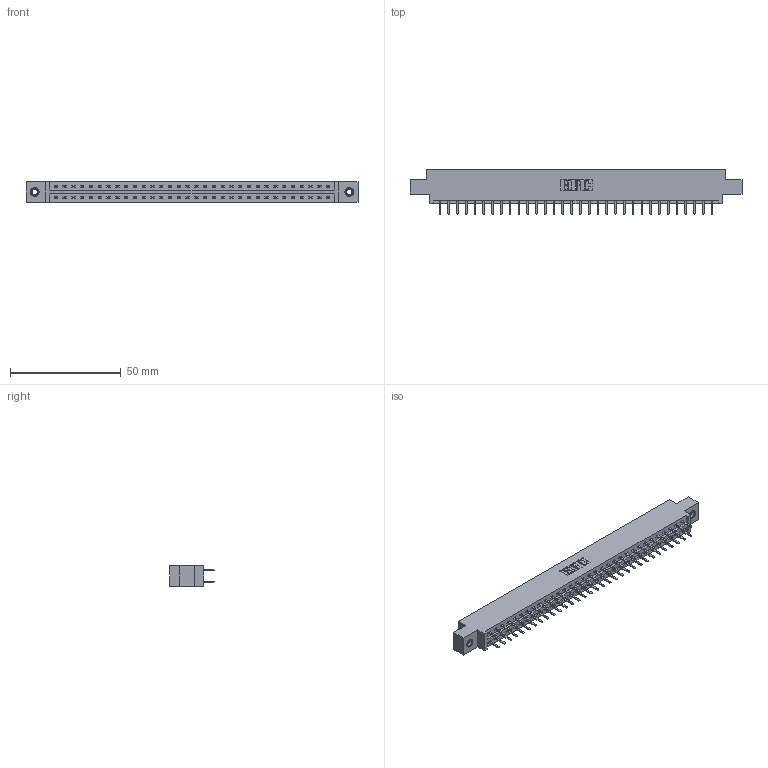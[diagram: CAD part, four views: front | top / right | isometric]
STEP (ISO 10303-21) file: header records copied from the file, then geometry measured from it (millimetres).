
FILE_DESCRIPTION (( 'STEP AP203' ), '1' );
FILE_NAME ('387-064-520-807.STEP', '2018-09-21T06:46:12', ( '' ), ( '' ), 'SwSTEP 2.0', 'SolidWorks 2016', '' );
FILE_SCHEMA (( 'CONFIG_CONTROL_DESIGN' ));
Length unit declared in the file: inch
Products named in the file (4): 345-250-001_345-250-005-103; 387-064-520-807; 337 Part_0.170 Offset - 0.156 Dia-TI; 345-292-001_345-293-120
Assembly tree (67 placements, depth 2):
  387-064-520-807
    337 Part_0.170 Offset - 0.156 Dia-TI
    345-292-001_345-293-120  x64
    345-250-001_345-250-005-103  x2
Bounding box: 149.81 x 20.02 x 9.4 mm (x, y, z)
Volume: 15495.8 mm3; surface area: 17484.4 mm2
Topology: 67 solids, 67 shells, 3890 faces, 11275 edges, 7338 vertices
Faces by surface type: plane 2666, cylinder 1208, cone 12, torus 4
Entity records: 27536 total; most frequent: CARTESIAN_POINT 4641, ORIENTED_EDGE 4558, DIRECTION 3985, EDGE_CURVE 2279, VECTOR 2127, LINE 2127, VERTEX_POINT 1512, AXIS2_PLACEMENT_3D 929
